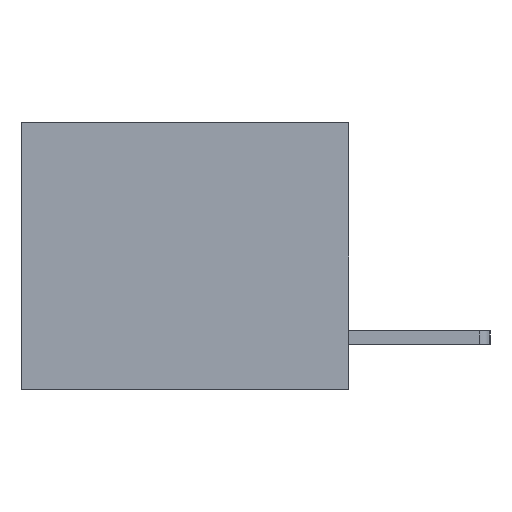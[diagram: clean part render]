
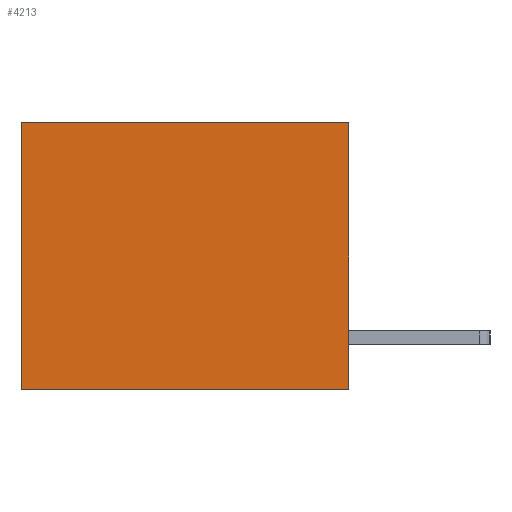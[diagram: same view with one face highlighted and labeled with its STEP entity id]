
A CAD part, left-side view. The second image highlights one B-rep face of the part: STEP entity #4213.
In plain terms, the highlighted planar face has unit normal (-1, 0, 0).
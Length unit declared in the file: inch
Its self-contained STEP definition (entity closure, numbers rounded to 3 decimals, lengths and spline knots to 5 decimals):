
#105 = VECTOR ( 'NONE', #6339, 39.37008 ) ;
#545 = VERTEX_POINT ( 'NONE', #6688 ) ;
#1051 = CARTESIAN_POINT ( 'NONE',  ( 0.3165, 0., -0.49 ) ) ;
#2957 = LINE ( 'NONE', #9744, #3619 ) ;
#2971 = CARTESIAN_POINT ( 'NONE',  ( 0.3165, 0.6, -0.49 ) ) ;
#3479 = CARTESIAN_POINT ( 'NONE',  ( 0.3165, 0., 0. ) ) ;
#3619 = VECTOR ( 'NONE', #5334, 39.37008 ) ;
#3653 = ORIENTED_EDGE ( 'NONE', *, *, #6896, .T. ) ;
#4213 = ADVANCED_FACE ( 'NONE', ( #8957 ), #13374, .F. ) ;
#4517 = VECTOR ( 'NONE', #13071, 39.37008 ) ;
#4769 = VERTEX_POINT ( 'NONE', #1051 ) ;
#4775 = CARTESIAN_POINT ( 'NONE',  ( 0.3165, 0.6, -0.49 ) ) ;
#5334 = DIRECTION ( 'NONE',  ( 0., 1., 0. ) ) ;
#6198 = LINE ( 'NONE', #3479, #4517 ) ;
#6339 = DIRECTION ( 'NONE',  ( 0., 0., -1. ) ) ;
#6565 = EDGE_LOOP ( 'NONE', ( #10346, #13256, #8201, #3653 ) ) ;
#6688 = CARTESIAN_POINT ( 'NONE',  ( 0.3165, 0., 0. ) ) ;
#6896 = EDGE_CURVE ( 'NONE', #545, #13648, #6198, .T. ) ;
#7139 = DIRECTION ( 'NONE',  ( 0., 0., -1. ) ) ;
#7468 = CARTESIAN_POINT ( 'NONE',  ( 0.3165, 0.6, 0. ) ) ;
#7590 = LINE ( 'NONE', #11470, #105 ) ;
#8201 = ORIENTED_EDGE ( 'NONE', *, *, #9821, .F. ) ;
#8957 = FACE_OUTER_BOUND ( 'NONE', #6565, .T. ) ;
#9017 = VECTOR ( 'NONE', #7139, 39.37008 ) ;
#9744 = CARTESIAN_POINT ( 'NONE',  ( 0.3165, 0., -0.49 ) ) ;
#9821 = EDGE_CURVE ( 'NONE', #545, #4769, #7590, .T. ) ;
#10333 = LINE ( 'NONE', #2971, #9017 ) ;
#10346 = ORIENTED_EDGE ( 'NONE', *, *, #12412, .T. ) ;
#11265 = VERTEX_POINT ( 'NONE', #4775 ) ;
#11470 = CARTESIAN_POINT ( 'NONE',  ( 0.3165, 0., -0.49 ) ) ;
#12273 = CARTESIAN_POINT ( 'NONE',  ( 0.3165, 0., -0.49 ) ) ;
#12412 = EDGE_CURVE ( 'NONE', #13648, #11265, #10333, .T. ) ;
#13071 = DIRECTION ( 'NONE',  ( 0., 1., 0. ) ) ;
#13256 = ORIENTED_EDGE ( 'NONE', *, *, #13589, .F. ) ;
#13286 = DIRECTION ( 'NONE',  ( 1., 0., 0. ) ) ;
#13374 = PLANE ( 'NONE',  #13751 ) ;
#13472 = DIRECTION ( 'NONE',  ( 0., 0., -1. ) ) ;
#13589 = EDGE_CURVE ( 'NONE', #4769, #11265, #2957, .T. ) ;
#13648 = VERTEX_POINT ( 'NONE', #7468 ) ;
#13751 = AXIS2_PLACEMENT_3D ( 'NONE', #12273, #13286, #13472 ) ;
